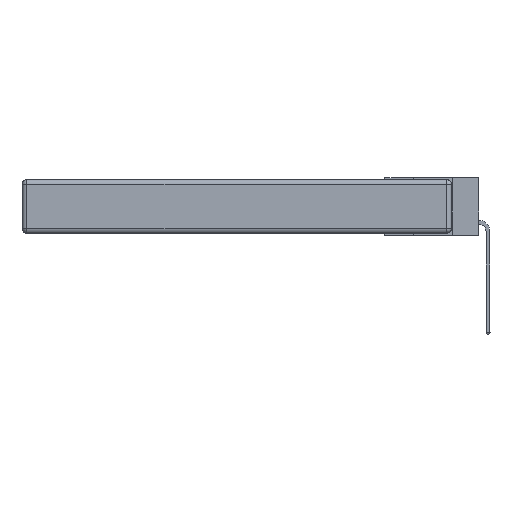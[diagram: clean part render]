
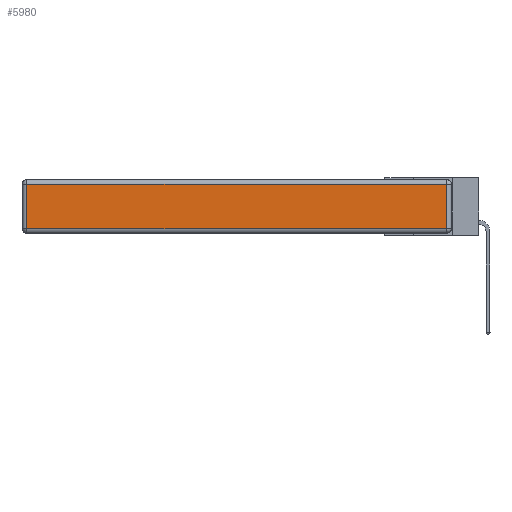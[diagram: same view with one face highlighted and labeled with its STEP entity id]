
A CAD part, left-side view. The second image highlights one B-rep face of the part: STEP entity #5980.
In plain terms, the highlighted planar face has unit normal (-1, 0, 0).
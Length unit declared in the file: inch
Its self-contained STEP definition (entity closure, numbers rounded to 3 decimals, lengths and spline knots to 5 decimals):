
#286 = CARTESIAN_POINT ( 'NONE',  ( 0., 2.72, -0.313 ) ) ;
#367 = EDGE_CURVE ( 'NONE', #26450, #11727, #28045, .T. ) ;
#535 = EDGE_LOOP ( 'NONE', ( #27206, #27368, #22230, #7922 ) ) ;
#2305 = PLANE ( 'NONE',  #21901 ) ;
#2342 = VERTEX_POINT ( 'NONE', #286 ) ;
#2438 = VECTOR ( 'NONE', #6370, 39.37008 ) ;
#3531 = DIRECTION ( 'NONE',  ( 0., 1., 0. ) ) ;
#3722 = DIRECTION ( 'NONE',  ( 0., 0., 1. ) ) ;
#4407 = FACE_OUTER_BOUND ( 'NONE', #535, .T. ) ;
#5980 = ADVANCED_FACE ( 'NONE', ( #4407 ), #2305, .T. ) ;
#6370 = DIRECTION ( 'NONE',  ( 0., 0., -1. ) ) ;
#6958 = DIRECTION ( 'NONE',  ( -1., 0., 0. ) ) ;
#7922 = ORIENTED_EDGE ( 'NONE', *, *, #18332, .T. ) ;
#8502 = CARTESIAN_POINT ( 'NONE',  ( 0., 0.03, -0.343 ) ) ;
#8889 = EDGE_CURVE ( 'NONE', #11727, #12744, #16394, .T. ) ;
#10160 = CARTESIAN_POINT ( 'NONE',  ( 0., 2.75, -0.03 ) ) ;
#10262 = EDGE_CURVE ( 'NONE', #2342, #26450, #18414, .T. ) ;
#10986 = CARTESIAN_POINT ( 'NONE',  ( 0., 0., -0.343 ) ) ;
#11727 = VERTEX_POINT ( 'NONE', #26211 ) ;
#12744 = VERTEX_POINT ( 'NONE', #15757 ) ;
#13676 = CARTESIAN_POINT ( 'NONE',  ( 0., 0., -0.313 ) ) ;
#14908 = LINE ( 'NONE', #21786, #2438 ) ;
#15698 = VECTOR ( 'NONE', #3531, 39.37008 ) ;
#15757 = CARTESIAN_POINT ( 'NONE',  ( 0., 2.72, -0.03 ) ) ;
#16394 = LINE ( 'NONE', #10160, #15698 ) ;
#18002 = VECTOR ( 'NONE', #3722, 39.37008 ) ;
#18332 = EDGE_CURVE ( 'NONE', #12744, #2342, #14908, .T. ) ;
#18414 = LINE ( 'NONE', #13676, #24564 ) ;
#21786 = CARTESIAN_POINT ( 'NONE',  ( 0., 2.72, -0.343 ) ) ;
#21901 = AXIS2_PLACEMENT_3D ( 'NONE', #10986, #6958, #26755 ) ;
#22230 = ORIENTED_EDGE ( 'NONE', *, *, #8889, .T. ) ;
#22232 = CARTESIAN_POINT ( 'NONE',  ( 0., 0.03, -0.313 ) ) ;
#24564 = VECTOR ( 'NONE', #27026, 39.37008 ) ;
#26211 = CARTESIAN_POINT ( 'NONE',  ( 0., 0.03, -0.03 ) ) ;
#26450 = VERTEX_POINT ( 'NONE', #22232 ) ;
#26755 = DIRECTION ( 'NONE',  ( 0., 0., 1. ) ) ;
#27026 = DIRECTION ( 'NONE',  ( 0., -1., 0. ) ) ;
#27206 = ORIENTED_EDGE ( 'NONE', *, *, #10262, .T. ) ;
#27368 = ORIENTED_EDGE ( 'NONE', *, *, #367, .T. ) ;
#28045 = LINE ( 'NONE', #8502, #18002 ) ;
